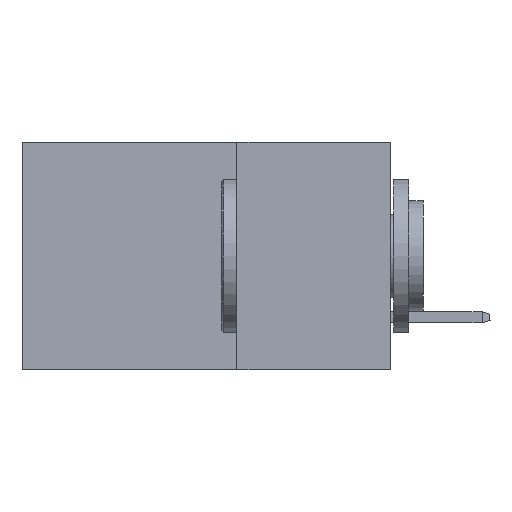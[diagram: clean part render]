
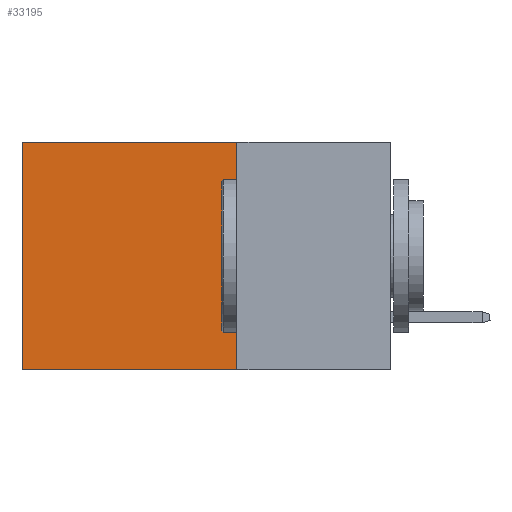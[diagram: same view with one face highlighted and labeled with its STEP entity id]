
A CAD part, left-side view. The second image highlights one B-rep face of the part: STEP entity #33195.
In plain terms, the highlighted planar face has unit normal (-1, 0, 0).
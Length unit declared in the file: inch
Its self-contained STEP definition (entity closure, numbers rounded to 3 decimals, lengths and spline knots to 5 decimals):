
#1288 = EDGE_CURVE ( 'NONE', #6105, #36213, #18762, .T. ) ;
#2172 = CARTESIAN_POINT ( 'NONE',  ( 0.2875, 0.25, -0.37 ) ) ;
#6037 = EDGE_LOOP ( 'NONE', ( #21422, #12027, #34873, #31944 ) ) ;
#6105 = VERTEX_POINT ( 'NONE', #12462 ) ;
#7504 = CARTESIAN_POINT ( 'NONE',  ( 0.2875, 0.25, 0. ) ) ;
#7521 = EDGE_CURVE ( 'NONE', #30813, #6105, #14209, .T. ) ;
#9046 = VECTOR ( 'NONE', #16534, 39.37008 ) ;
#11055 = VECTOR ( 'NONE', #37003, 39.37008 ) ;
#12027 = ORIENTED_EDGE ( 'NONE', *, *, #1288, .F. ) ;
#12370 = DIRECTION ( 'NONE',  ( 1., 0., 0. ) ) ;
#12462 = CARTESIAN_POINT ( 'NONE',  ( 0.2875, 0.25, -0.37 ) ) ;
#13838 = LINE ( 'NONE', #30794, #11055 ) ;
#14209 = LINE ( 'NONE', #33650, #37007 ) ;
#16534 = DIRECTION ( 'NONE',  ( 0., 0., -1. ) ) ;
#18247 = PLANE ( 'NONE',  #24027 ) ;
#18762 = LINE ( 'NONE', #2172, #29485 ) ;
#19272 = CARTESIAN_POINT ( 'NONE',  ( 0.2875, 0.6, 0. ) ) ;
#20695 = CARTESIAN_POINT ( 'NONE',  ( 0.2875, 0.6, -0.37 ) ) ;
#21225 = EDGE_CURVE ( 'NONE', #30813, #36366, #13838, .T. ) ;
#21422 = ORIENTED_EDGE ( 'NONE', *, *, #23744, .T. ) ;
#21696 = DIRECTION ( 'NONE',  ( 0., 0., -1. ) ) ;
#23744 = EDGE_CURVE ( 'NONE', #36366, #36213, #24838, .T. ) ;
#23753 = FACE_OUTER_BOUND ( 'NONE', #6037, .T. ) ;
#24027 = AXIS2_PLACEMENT_3D ( 'NONE', #27201, #12370, #36138 ) ;
#24838 = LINE ( 'NONE', #19272, #9046 ) ;
#25961 = DIRECTION ( 'NONE',  ( 0., 1., 0. ) ) ;
#27201 = CARTESIAN_POINT ( 'NONE',  ( 0.2875, 0.25, 0. ) ) ;
#29485 = VECTOR ( 'NONE', #25961, 39.37008 ) ;
#30794 = CARTESIAN_POINT ( 'NONE',  ( 0.2875, 0.25, 0. ) ) ;
#30813 = VERTEX_POINT ( 'NONE', #7504 ) ;
#31944 = ORIENTED_EDGE ( 'NONE', *, *, #21225, .T. ) ;
#32679 = CARTESIAN_POINT ( 'NONE',  ( 0.2875, 0.6, 0. ) ) ;
#33195 = ADVANCED_FACE ( 'NONE', ( #23753 ), #18247, .F. ) ;
#33650 = CARTESIAN_POINT ( 'NONE',  ( 0.2875, 0.25, 0. ) ) ;
#34873 = ORIENTED_EDGE ( 'NONE', *, *, #7521, .F. ) ;
#36138 = DIRECTION ( 'NONE',  ( 0., 0., -1. ) ) ;
#36213 = VERTEX_POINT ( 'NONE', #20695 ) ;
#36366 = VERTEX_POINT ( 'NONE', #32679 ) ;
#37003 = DIRECTION ( 'NONE',  ( 0., 1., 0. ) ) ;
#37007 = VECTOR ( 'NONE', #21696, 39.37008 ) ;
